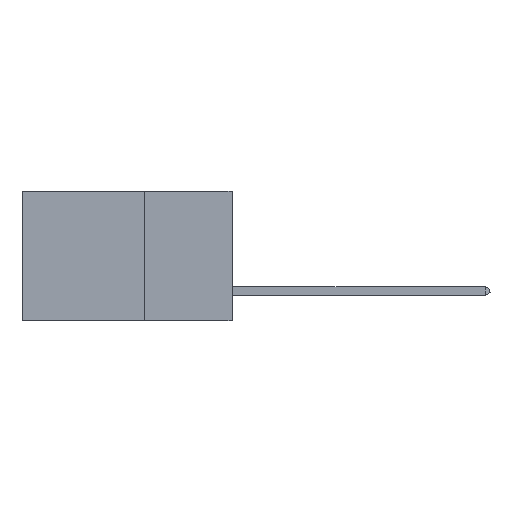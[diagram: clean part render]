
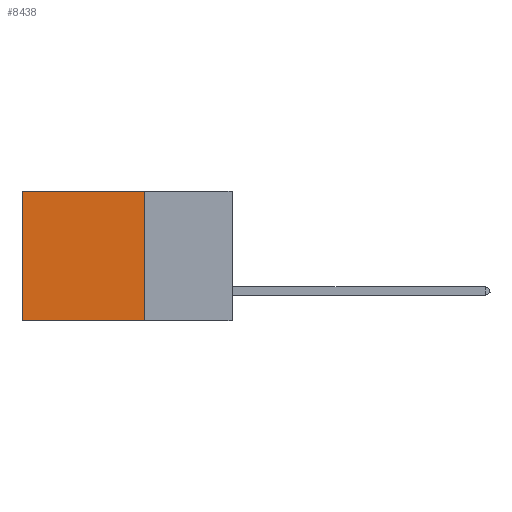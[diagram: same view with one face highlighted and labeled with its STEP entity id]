
A CAD part, left-side view. The second image highlights one B-rep face of the part: STEP entity #8438.
In plain terms, the highlighted planar face has unit normal (-1, 0, 0).
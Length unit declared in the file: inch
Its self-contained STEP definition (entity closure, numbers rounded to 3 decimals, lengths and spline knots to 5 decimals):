
#110 = EDGE_CURVE ( 'NONE', #17497, #591, #12686, .T. ) ;
#508 = VECTOR ( 'NONE', #9029, 39.37008 ) ;
#591 = VERTEX_POINT ( 'NONE', #11405 ) ;
#769 = CARTESIAN_POINT ( 'NONE',  ( 0.2875, 0.6, 0. ) ) ;
#1368 = DIRECTION ( 'NONE',  ( 0., 0., -1. ) ) ;
#1605 = FACE_OUTER_BOUND ( 'NONE', #2734, .T. ) ;
#2734 = EDGE_LOOP ( 'NONE', ( #6246, #10311, #6148, #6032 ) ) ;
#2878 = CARTESIAN_POINT ( 'NONE',  ( 0.2875, 0.25, 0. ) ) ;
#3267 = LINE ( 'NONE', #15418, #15661 ) ;
#4022 = DIRECTION ( 'NONE',  ( 0., 1., 0. ) ) ;
#5923 = CARTESIAN_POINT ( 'NONE',  ( 0.2875, 0.25, 0. ) ) ;
#6032 = ORIENTED_EDGE ( 'NONE', *, *, #6600, .T. ) ;
#6148 = ORIENTED_EDGE ( 'NONE', *, *, #10460, .F. ) ;
#6246 = ORIENTED_EDGE ( 'NONE', *, *, #110, .T. ) ;
#6261 = DIRECTION ( 'NONE',  ( 1., 0., 0. ) ) ;
#6600 = EDGE_CURVE ( 'NONE', #17080, #17497, #18874, .T. ) ;
#6732 = DIRECTION ( 'NONE',  ( 0., 0., -1. ) ) ;
#7732 = PLANE ( 'NONE',  #17109 ) ;
#8438 = ADVANCED_FACE ( 'NONE', ( #1605 ), #7732, .F. ) ;
#9029 = DIRECTION ( 'NONE',  ( 0., 0., -1. ) ) ;
#10311 = ORIENTED_EDGE ( 'NONE', *, *, #11447, .F. ) ;
#10352 = LINE ( 'NONE', #5923, #508 ) ;
#10460 = EDGE_CURVE ( 'NONE', #17080, #20049, #10352, .T. ) ;
#10859 = DIRECTION ( 'NONE',  ( 0., 1., 0. ) ) ;
#11139 = CARTESIAN_POINT ( 'NONE',  ( 0.2875, 0.25, 0. ) ) ;
#11405 = CARTESIAN_POINT ( 'NONE',  ( 0.2875, 0.6, -0.37 ) ) ;
#11447 = EDGE_CURVE ( 'NONE', #20049, #591, #3267, .T. ) ;
#12450 = CARTESIAN_POINT ( 'NONE',  ( 0.2875, 0.25, -0.37 ) ) ;
#12686 = LINE ( 'NONE', #14017, #18270 ) ;
#14017 = CARTESIAN_POINT ( 'NONE',  ( 0.2875, 0.6, 0. ) ) ;
#15370 = VECTOR ( 'NONE', #10859, 39.37008 ) ;
#15418 = CARTESIAN_POINT ( 'NONE',  ( 0.2875, 0.25, -0.37 ) ) ;
#15661 = VECTOR ( 'NONE', #4022, 39.37008 ) ;
#17080 = VERTEX_POINT ( 'NONE', #11139 ) ;
#17109 = AXIS2_PLACEMENT_3D ( 'NONE', #2878, #6261, #1368 ) ;
#17497 = VERTEX_POINT ( 'NONE', #769 ) ;
#18270 = VECTOR ( 'NONE', #6732, 39.37008 ) ;
#18874 = LINE ( 'NONE', #20474, #15370 ) ;
#20049 = VERTEX_POINT ( 'NONE', #12450 ) ;
#20474 = CARTESIAN_POINT ( 'NONE',  ( 0.2875, 0.25, 0. ) ) ;
